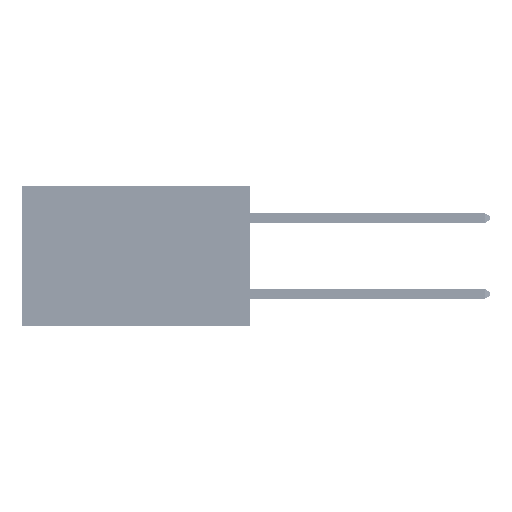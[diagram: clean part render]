
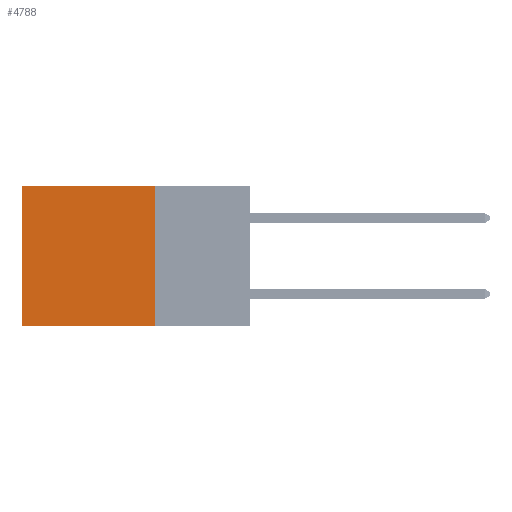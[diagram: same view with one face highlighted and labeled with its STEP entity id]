
A CAD part, left-side view. The second image highlights one B-rep face of the part: STEP entity #4788.
In plain terms, the highlighted planar face has unit normal (-1, 0, 0).
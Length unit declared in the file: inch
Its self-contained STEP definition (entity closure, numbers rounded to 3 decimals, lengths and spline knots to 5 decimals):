
#894 = VECTOR ( 'NONE', #20037, 39.37008 ) ;
#1081 = DIRECTION ( 'NONE',  ( 0., 1., 0. ) ) ;
#1565 = CARTESIAN_POINT ( 'NONE',  ( 0.2875, 0.25, -0.37 ) ) ;
#1895 = LINE ( 'NONE', #38901, #8446 ) ;
#3836 = LINE ( 'NONE', #23184, #38864 ) ;
#4705 = FACE_OUTER_BOUND ( 'NONE', #16498, .T. ) ;
#4788 = ADVANCED_FACE ( 'NONE', ( #4705 ), #31402, .F. ) ;
#5097 = LINE ( 'NONE', #5573, #894 ) ;
#5573 = CARTESIAN_POINT ( 'NONE',  ( 0.2875, 0.6, 0. ) ) ;
#6461 = CARTESIAN_POINT ( 'NONE',  ( 0.2875, 0.6, 0. ) ) ;
#8446 = VECTOR ( 'NONE', #30586, 39.37008 ) ;
#9071 = ORIENTED_EDGE ( 'NONE', *, *, #22947, .F. ) ;
#11058 = CARTESIAN_POINT ( 'NONE',  ( 0.2875, 0.25, -0.37 ) ) ;
#12162 = DIRECTION ( 'NONE',  ( 0., 0., -1. ) ) ;
#15568 = EDGE_CURVE ( 'NONE', #45413, #42307, #5097, .T. ) ;
#15981 = VERTEX_POINT ( 'NONE', #40026 ) ;
#16498 = EDGE_LOOP ( 'NONE', ( #25004, #9071, #45770, #47971 ) ) ;
#16615 = AXIS2_PLACEMENT_3D ( 'NONE', #34818, #39223, #23340 ) ;
#17155 = EDGE_CURVE ( 'NONE', #15981, #19227, #3836, .T. ) ;
#19227 = VERTEX_POINT ( 'NONE', #11058 ) ;
#20037 = DIRECTION ( 'NONE',  ( 0., 0., -1. ) ) ;
#21233 = EDGE_CURVE ( 'NONE', #15981, #45413, #1895, .T. ) ;
#22947 = EDGE_CURVE ( 'NONE', #19227, #42307, #34400, .T. ) ;
#23184 = CARTESIAN_POINT ( 'NONE',  ( 0.2875, 0.25, 0. ) ) ;
#23340 = DIRECTION ( 'NONE',  ( 0., 0., -1. ) ) ;
#25004 = ORIENTED_EDGE ( 'NONE', *, *, #15568, .T. ) ;
#30586 = DIRECTION ( 'NONE',  ( 0., 1., 0. ) ) ;
#31402 = PLANE ( 'NONE',  #16615 ) ;
#34400 = LINE ( 'NONE', #1565, #40712 ) ;
#34818 = CARTESIAN_POINT ( 'NONE',  ( 0.2875, 0.25, 0. ) ) ;
#38864 = VECTOR ( 'NONE', #12162, 39.37008 ) ;
#38901 = CARTESIAN_POINT ( 'NONE',  ( 0.2875, 0.25, 0. ) ) ;
#39223 = DIRECTION ( 'NONE',  ( 1., 0., 0. ) ) ;
#40026 = CARTESIAN_POINT ( 'NONE',  ( 0.2875, 0.25, 0. ) ) ;
#40712 = VECTOR ( 'NONE', #1081, 39.37008 ) ;
#42307 = VERTEX_POINT ( 'NONE', #43463 ) ;
#43463 = CARTESIAN_POINT ( 'NONE',  ( 0.2875, 0.6, -0.37 ) ) ;
#45413 = VERTEX_POINT ( 'NONE', #6461 ) ;
#45770 = ORIENTED_EDGE ( 'NONE', *, *, #17155, .F. ) ;
#47971 = ORIENTED_EDGE ( 'NONE', *, *, #21233, .T. ) ;
